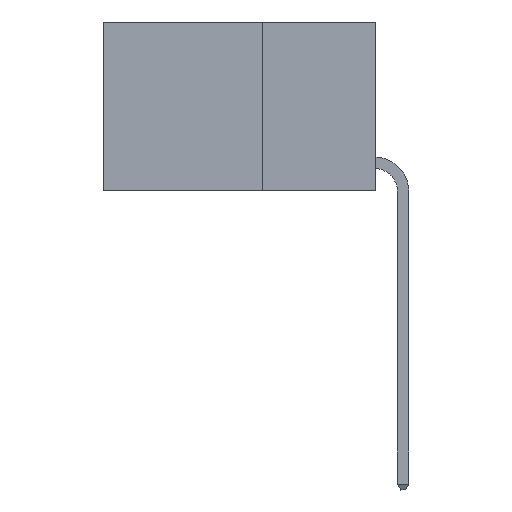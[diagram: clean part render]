
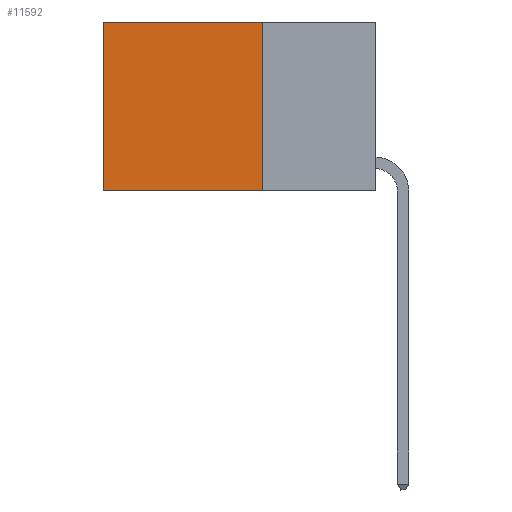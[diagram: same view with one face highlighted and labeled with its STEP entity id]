
A CAD part, left-side view. The second image highlights one B-rep face of the part: STEP entity #11592.
In plain terms, the highlighted planar face has unit normal (-1, 0, 0).
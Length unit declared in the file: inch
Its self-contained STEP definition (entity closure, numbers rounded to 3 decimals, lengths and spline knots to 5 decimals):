
#879 = VERTEX_POINT ( 'NONE', #4486 ) ;
#938 = EDGE_CURVE ( 'NONE', #4543, #879, #1438, .T. ) ;
#1438 = LINE ( 'NONE', #3952, #3004 ) ;
#1864 = DIRECTION ( 'NONE',  ( 0., 1., 0. ) ) ;
#2686 = VERTEX_POINT ( 'NONE', #14217 ) ;
#2754 = DIRECTION ( 'NONE',  ( 0., 0., -1. ) ) ;
#2854 = LINE ( 'NONE', #12442, #13130 ) ;
#2999 = DIRECTION ( 'NONE',  ( 0., 0., -1. ) ) ;
#3004 = VECTOR ( 'NONE', #9444, 39.37008 ) ;
#3952 = CARTESIAN_POINT ( 'NONE',  ( 0.2625, 0.6, 0. ) ) ;
#4019 = CARTESIAN_POINT ( 'NONE',  ( 0.2625, 0.25, 0. ) ) ;
#4486 = CARTESIAN_POINT ( 'NONE',  ( 0.2625, 0.6, -0.37 ) ) ;
#4543 = VERTEX_POINT ( 'NONE', #15347 ) ;
#4976 = VECTOR ( 'NONE', #1864, 39.37008 ) ;
#6698 = AXIS2_PLACEMENT_3D ( 'NONE', #4019, #7101, #2754 ) ;
#6987 = EDGE_CURVE ( 'NONE', #2686, #4543, #15949, .T. ) ;
#6999 = FACE_OUTER_BOUND ( 'NONE', #9915, .T. ) ;
#7101 = DIRECTION ( 'NONE',  ( 1., 0., 0. ) ) ;
#7167 = LINE ( 'NONE', #13681, #10193 ) ;
#7376 = DIRECTION ( 'NONE',  ( 0., 1., 0. ) ) ;
#7541 = CARTESIAN_POINT ( 'NONE',  ( 0.2625, 0.25, 0. ) ) ;
#8774 = ORIENTED_EDGE ( 'NONE', *, *, #6987, .T. ) ;
#9152 = ORIENTED_EDGE ( 'NONE', *, *, #938, .T. ) ;
#9444 = DIRECTION ( 'NONE',  ( 0., 0., -1. ) ) ;
#9665 = EDGE_CURVE ( 'NONE', #11604, #879, #2854, .T. ) ;
#9702 = PLANE ( 'NONE',  #6698 ) ;
#9915 = EDGE_LOOP ( 'NONE', ( #9152, #12186, #11093, #8774 ) ) ;
#10193 = VECTOR ( 'NONE', #2999, 39.37008 ) ;
#11093 = ORIENTED_EDGE ( 'NONE', *, *, #14633, .F. ) ;
#11592 = ADVANCED_FACE ( 'NONE', ( #6999 ), #9702, .F. ) ;
#11604 = VERTEX_POINT ( 'NONE', #15304 ) ;
#12186 = ORIENTED_EDGE ( 'NONE', *, *, #9665, .F. ) ;
#12442 = CARTESIAN_POINT ( 'NONE',  ( 0.2625, 0.25, -0.37 ) ) ;
#13130 = VECTOR ( 'NONE', #7376, 39.37008 ) ;
#13681 = CARTESIAN_POINT ( 'NONE',  ( 0.2625, 0.25, 0. ) ) ;
#14217 = CARTESIAN_POINT ( 'NONE',  ( 0.2625, 0.25, 0. ) ) ;
#14633 = EDGE_CURVE ( 'NONE', #2686, #11604, #7167, .T. ) ;
#15304 = CARTESIAN_POINT ( 'NONE',  ( 0.2625, 0.25, -0.37 ) ) ;
#15347 = CARTESIAN_POINT ( 'NONE',  ( 0.2625, 0.6, 0. ) ) ;
#15949 = LINE ( 'NONE', #7541, #4976 ) ;
